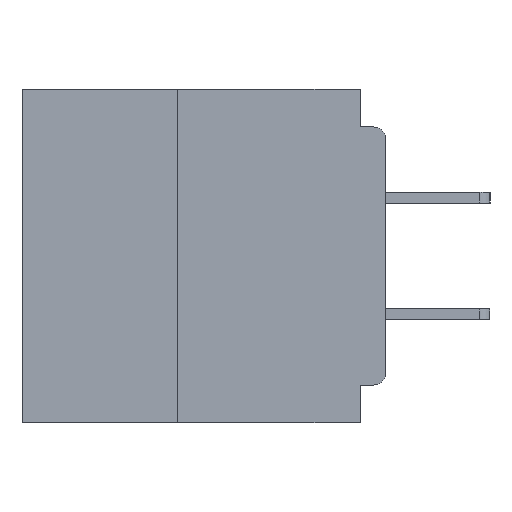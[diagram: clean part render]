
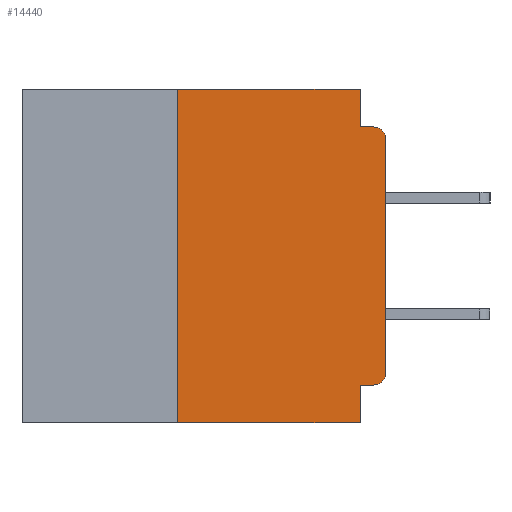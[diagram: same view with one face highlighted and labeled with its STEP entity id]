
A CAD part, left-side view. The second image highlights one B-rep face of the part: STEP entity #14440.
In plain terms, the highlighted planar face has unit normal (-1, 0, 0).
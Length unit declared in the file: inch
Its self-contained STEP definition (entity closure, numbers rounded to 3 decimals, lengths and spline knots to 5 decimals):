
#280 = CARTESIAN_POINT ( 'NONE',  ( 0., 0.031, 0. ) ) ;
#497 = DIRECTION ( 'NONE',  ( 0., -1., 0. ) ) ;
#582 = CARTESIAN_POINT ( 'NONE',  ( 0., 0.031, 0. ) ) ;
#880 = CARTESIAN_POINT ( 'NONE',  ( 0., 0.031, -0.4 ) ) ;
#1741 = LINE ( 'NONE', #21109, #27485 ) ;
#2511 = LINE ( 'NONE', #35563, #27202 ) ;
#2732 = CARTESIAN_POINT ( 'NONE',  ( 0., 0.25, 0. ) ) ;
#2795 = CARTESIAN_POINT ( 'NONE',  ( 0., 0.015, -0.355 ) ) ;
#3822 = AXIS2_PLACEMENT_3D ( 'NONE', #32594, #12468, #35951 ) ;
#3959 = DIRECTION ( 'NONE',  ( 0., 0., -1. ) ) ;
#3989 = CARTESIAN_POINT ( 'NONE',  ( 0., 0.015, -0.34 ) ) ;
#4083 = CARTESIAN_POINT ( 'NONE',  ( 0., 0., -0.06 ) ) ;
#5741 = VERTEX_POINT ( 'NONE', #38350 ) ;
#5770 = LINE ( 'NONE', #880, #31498 ) ;
#6438 = CARTESIAN_POINT ( 'NONE',  ( 0., 0., -0.045 ) ) ;
#6457 = VECTOR ( 'NONE', #18702, 39.37008 ) ;
#6828 = ORIENTED_EDGE ( 'NONE', *, *, #26771, .F. ) ;
#7216 = EDGE_CURVE ( 'NONE', #25973, #27376, #2511, .T. ) ;
#7374 = DIRECTION ( 'NONE',  ( 0., 0., -1. ) ) ;
#7869 = VERTEX_POINT ( 'NONE', #12020 ) ;
#7877 = AXIS2_PLACEMENT_3D ( 'NONE', #13133, #36746, #16661 ) ;
#8251 = EDGE_CURVE ( 'NONE', #34791, #21754, #19197, .T. ) ;
#9753 = DIRECTION ( 'NONE',  ( 0., -1., 0. ) ) ;
#9782 = VERTEX_POINT ( 'NONE', #2795 ) ;
#9984 = EDGE_CURVE ( 'NONE', #9782, #25973, #43176, .T. ) ;
#10269 = VECTOR ( 'NONE', #3959, 39.37008 ) ;
#10738 = EDGE_CURVE ( 'NONE', #5741, #21206, #41565, .T. ) ;
#10898 = EDGE_CURVE ( 'NONE', #21206, #34791, #42048, .T. ) ;
#11864 = ORIENTED_EDGE ( 'NONE', *, *, #7216, .T. ) ;
#12020 = CARTESIAN_POINT ( 'NONE',  ( 0., 0.031, -0.4 ) ) ;
#12468 = DIRECTION ( 'NONE',  ( -1., 0., 0. ) ) ;
#13133 = CARTESIAN_POINT ( 'NONE',  ( 0., 0.437, 0. ) ) ;
#14007 = VECTOR ( 'NONE', #9753, 39.37008 ) ;
#14440 = ADVANCED_FACE ( 'NONE', ( #41254 ), #19874, .F. ) ;
#15225 = ORIENTED_EDGE ( 'NONE', *, *, #43338, .F. ) ;
#15760 = CARTESIAN_POINT ( 'NONE',  ( 0., 0., -0.34 ) ) ;
#15908 = CARTESIAN_POINT ( 'NONE',  ( 0., 0.031, -0.045 ) ) ;
#16381 = ORIENTED_EDGE ( 'NONE', *, *, #10738, .F. ) ;
#16661 = DIRECTION ( 'NONE',  ( 0., 0., -1. ) ) ;
#16827 = ORIENTED_EDGE ( 'NONE', *, *, #9984, .T. ) ;
#17055 = ORIENTED_EDGE ( 'NONE', *, *, #35418, .T. ) ;
#17205 = CARTESIAN_POINT ( 'NONE',  ( 0., 0.437, -0.4 ) ) ;
#18702 = DIRECTION ( 'NONE',  ( 0., -1., 0. ) ) ;
#18818 = DIRECTION ( 'NONE',  ( 0., 0., 1. ) ) ;
#19197 = LINE ( 'NONE', #582, #10269 ) ;
#19874 = PLANE ( 'NONE',  #7877 ) ;
#20388 = LINE ( 'NONE', #17205, #29297 ) ;
#20483 = CIRCLE ( 'NONE', #3822, 0.015 ) ;
#21109 = CARTESIAN_POINT ( 'NONE',  ( 0., 0., -0.355 ) ) ;
#21194 = CARTESIAN_POINT ( 'NONE',  ( 0., 0.25, -0.4 ) ) ;
#21206 = VERTEX_POINT ( 'NONE', #2732 ) ;
#21754 = VERTEX_POINT ( 'NONE', #15908 ) ;
#22727 = ORIENTED_EDGE ( 'NONE', *, *, #10898, .F. ) ;
#23729 = VECTOR ( 'NONE', #41287, 39.37008 ) ;
#25422 = CARTESIAN_POINT ( 'NONE',  ( 0., 0.437, 0. ) ) ;
#25973 = VERTEX_POINT ( 'NONE', #15760 ) ;
#26771 = EDGE_CURVE ( 'NONE', #9782, #28785, #1741, .T. ) ;
#27202 = VECTOR ( 'NONE', #18818, 39.37008 ) ;
#27350 = EDGE_LOOP ( 'NONE', ( #11864, #41689, #41097, #34607, #22727, #16381, #17055, #15225, #6828, #16827 ) ) ;
#27376 = VERTEX_POINT ( 'NONE', #4083 ) ;
#27460 = DIRECTION ( 'NONE',  ( -1., 0., 0. ) ) ;
#27485 = VECTOR ( 'NONE', #34650, 39.37008 ) ;
#28137 = CARTESIAN_POINT ( 'NONE',  ( 0., 0.031, -0.355 ) ) ;
#28785 = VERTEX_POINT ( 'NONE', #28137 ) ;
#29297 = VECTOR ( 'NONE', #497, 39.37008 ) ;
#29670 = VERTEX_POINT ( 'NONE', #38145 ) ;
#30972 = DIRECTION ( 'NONE',  ( 0., 0., -1. ) ) ;
#31498 = VECTOR ( 'NONE', #30972, 39.37008 ) ;
#32594 = CARTESIAN_POINT ( 'NONE',  ( 0., 0.015, -0.06 ) ) ;
#34607 = ORIENTED_EDGE ( 'NONE', *, *, #8251, .F. ) ;
#34650 = DIRECTION ( 'NONE',  ( 0., 1., 0. ) ) ;
#34737 = AXIS2_PLACEMENT_3D ( 'NONE', #3989, #27460, #7374 ) ;
#34791 = VERTEX_POINT ( 'NONE', #280 ) ;
#35418 = EDGE_CURVE ( 'NONE', #5741, #7869, #20388, .T. ) ;
#35563 = CARTESIAN_POINT ( 'NONE',  ( 0., 0., 0. ) ) ;
#35951 = DIRECTION ( 'NONE',  ( 0., 0., -1. ) ) ;
#36423 = EDGE_CURVE ( 'NONE', #21754, #29670, #40737, .T. ) ;
#36746 = DIRECTION ( 'NONE',  ( 1., 0., 0. ) ) ;
#38145 = CARTESIAN_POINT ( 'NONE',  ( 0., 0.015, -0.045 ) ) ;
#38350 = CARTESIAN_POINT ( 'NONE',  ( 0., 0.25, -0.4 ) ) ;
#40737 = LINE ( 'NONE', #6438, #14007 ) ;
#41097 = ORIENTED_EDGE ( 'NONE', *, *, #36423, .F. ) ;
#41254 = FACE_OUTER_BOUND ( 'NONE', #27350, .T. ) ;
#41287 = DIRECTION ( 'NONE',  ( 0., 0., 1. ) ) ;
#41565 = LINE ( 'NONE', #21194, #23729 ) ;
#41689 = ORIENTED_EDGE ( 'NONE', *, *, #42965, .T. ) ;
#42048 = LINE ( 'NONE', #25422, #6457 ) ;
#42965 = EDGE_CURVE ( 'NONE', #27376, #29670, #20483, .T. ) ;
#43176 = CIRCLE ( 'NONE', #34737, 0.015 ) ;
#43338 = EDGE_CURVE ( 'NONE', #28785, #7869, #5770, .T. ) ;
